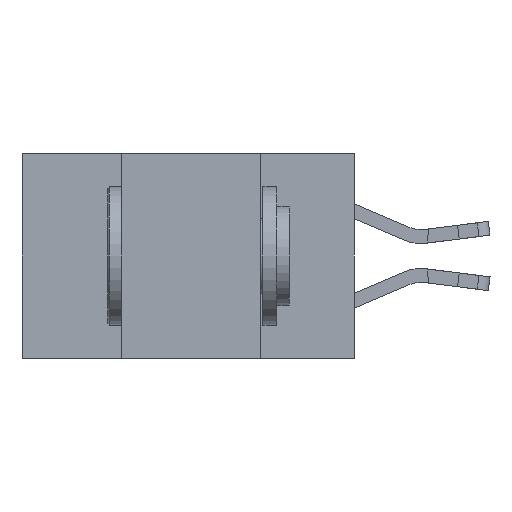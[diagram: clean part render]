
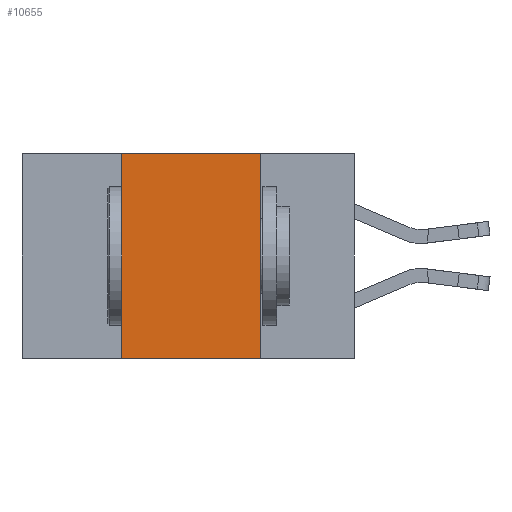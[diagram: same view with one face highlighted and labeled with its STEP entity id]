
A CAD part, left-side view. The second image highlights one B-rep face of the part: STEP entity #10655.
In plain terms, the highlighted planar face has unit normal (-1, 0, 0).
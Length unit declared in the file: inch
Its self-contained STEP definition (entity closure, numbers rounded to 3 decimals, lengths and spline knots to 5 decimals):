
#132 = VERTEX_POINT ( 'NONE', #6854 ) ;
#181 = ORIENTED_EDGE ( 'NONE', *, *, #1486, .T. ) ;
#558 = VERTEX_POINT ( 'NONE', #2384 ) ;
#574 = EDGE_CURVE ( 'NONE', #132, #700, #9070, .T. ) ;
#700 = VERTEX_POINT ( 'NONE', #981 ) ;
#727 = CARTESIAN_POINT ( 'NONE',  ( 0., 0.6, -0.37 ) ) ;
#810 = CARTESIAN_POINT ( 'NONE',  ( 0., 0.6, 0. ) ) ;
#981 = CARTESIAN_POINT ( 'NONE',  ( 0., 0.17, 0. ) ) ;
#1327 = VECTOR ( 'NONE', #4211, 39.37008 ) ;
#1486 = EDGE_CURVE ( 'NONE', #4911, #558, #9011, .T. ) ;
#2004 = LINE ( 'NONE', #9958, #8785 ) ;
#2014 = LINE ( 'NONE', #7897, #1327 ) ;
#2030 = VECTOR ( 'NONE', #4226, 39.37008 ) ;
#2384 = CARTESIAN_POINT ( 'NONE',  ( 0., 0.17, -0.37 ) ) ;
#2657 = DIRECTION ( 'NONE',  ( 1., 0., 0. ) ) ;
#4184 = PLANE ( 'NONE',  #5482 ) ;
#4211 = DIRECTION ( 'NONE',  ( 0., 0., 1. ) ) ;
#4226 = DIRECTION ( 'NONE',  ( 0., -1., 0. ) ) ;
#4911 = VERTEX_POINT ( 'NONE', #10764 ) ;
#5482 = AXIS2_PLACEMENT_3D ( 'NONE', #810, #2657, #5969 ) ;
#5607 = ORIENTED_EDGE ( 'NONE', *, *, #574, .F. ) ;
#5892 = CARTESIAN_POINT ( 'NONE',  ( 0., 0.6, 0. ) ) ;
#5916 = ORIENTED_EDGE ( 'NONE', *, *, #9014, .F. ) ;
#5969 = DIRECTION ( 'NONE',  ( 0., 0., -1. ) ) ;
#6256 = DIRECTION ( 'NONE',  ( 0., 0., -1. ) ) ;
#6801 = DIRECTION ( 'NONE',  ( 0., -1., 0. ) ) ;
#6854 = CARTESIAN_POINT ( 'NONE',  ( 0., 0.42, 0. ) ) ;
#6988 = FACE_OUTER_BOUND ( 'NONE', #10384, .T. ) ;
#7362 = ORIENTED_EDGE ( 'NONE', *, *, #8258, .F. ) ;
#7897 = CARTESIAN_POINT ( 'NONE',  ( 0., 0.42, -0.37 ) ) ;
#8258 = EDGE_CURVE ( 'NONE', #4911, #132, #2014, .T. ) ;
#8785 = VECTOR ( 'NONE', #6256, 39.37008 ) ;
#9011 = LINE ( 'NONE', #727, #9932 ) ;
#9014 = EDGE_CURVE ( 'NONE', #700, #558, #2004, .T. ) ;
#9070 = LINE ( 'NONE', #5892, #2030 ) ;
#9932 = VECTOR ( 'NONE', #6801, 39.37008 ) ;
#9958 = CARTESIAN_POINT ( 'NONE',  ( 0., 0.17, -0.37 ) ) ;
#10384 = EDGE_LOOP ( 'NONE', ( #5916, #5607, #7362, #181 ) ) ;
#10655 = ADVANCED_FACE ( 'NONE', ( #6988 ), #4184, .F. ) ;
#10764 = CARTESIAN_POINT ( 'NONE',  ( 0., 0.42, -0.37 ) ) ;
